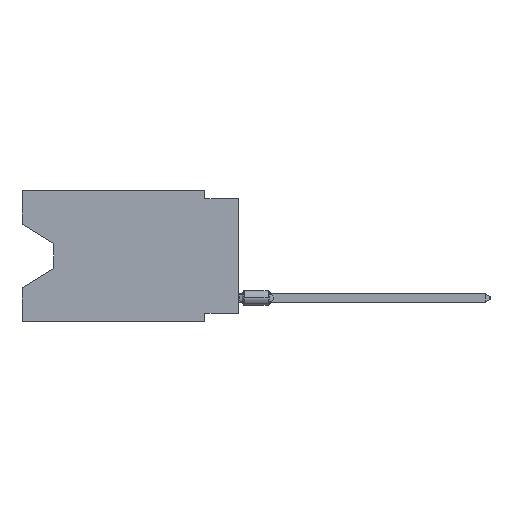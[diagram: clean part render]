
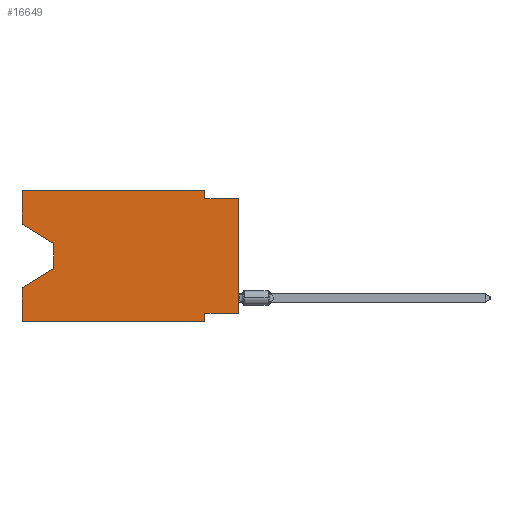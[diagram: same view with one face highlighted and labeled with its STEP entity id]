
A CAD part, left-side view. The second image highlights one B-rep face of the part: STEP entity #16649.
In plain terms, the highlighted planar face has unit normal (-1, 0, 0).
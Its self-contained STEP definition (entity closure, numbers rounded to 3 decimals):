
#107 = VERTEX_POINT ( 'NONE', #27007 ) ;
#235 = LINE ( 'NONE', #24681, #61684 ) ;
#474 = DIRECTION ( 'NONE',  ( 1., 0., 0. ) ) ;
#964 = CARTESIAN_POINT ( 'NONE',  ( 0., 0., -9.271 ) ) ;
#1285 = VERTEX_POINT ( 'NONE', #38073 ) ;
#1314 = EDGE_CURVE ( 'NONE', #22827, #63308, #53799, .T. ) ;
#1412 = CARTESIAN_POINT ( 'NONE',  ( 0., 16.383, 0. ) ) ;
#2039 = ORIENTED_EDGE ( 'NONE', *, *, #60994, .T. ) ;
#2714 = VECTOR ( 'NONE', #15578, 1000. ) ;
#4916 = CARTESIAN_POINT ( 'NONE',  ( 0., 0., -9.271 ) ) ;
#5628 = LINE ( 'NONE', #35447, #20235 ) ;
#5804 = ORIENTED_EDGE ( 'NONE', *, *, #1314, .F. ) ;
#6090 = LINE ( 'NONE', #1412, #43253 ) ;
#6978 = LINE ( 'NONE', #964, #58350 ) ;
#8796 = ORIENTED_EDGE ( 'NONE', *, *, #17196, .T. ) ;
#9389 = CARTESIAN_POINT ( 'NONE',  ( 0., 13.97, -4.013 ) ) ;
#9947 = DIRECTION ( 'NONE',  ( 0., 0., 1. ) ) ;
#9989 = DIRECTION ( 'NONE',  ( 0., 0., 1. ) ) ;
#10262 = LINE ( 'NONE', #55491, #43529 ) ;
#10268 = CARTESIAN_POINT ( 'NONE',  ( 0., 16.383, -9.906 ) ) ;
#10879 = CARTESIAN_POINT ( 'NONE',  ( 0., 16.383, -2.546 ) ) ;
#11327 = DIRECTION ( 'NONE',  ( 0., 1., 0. ) ) ;
#11520 = DIRECTION ( 'NONE',  ( 0., 0., -1. ) ) ;
#14663 = DIRECTION ( 'NONE',  ( 0., 0.855, -0.519 ) ) ;
#15171 = ORIENTED_EDGE ( 'NONE', *, *, #45111, .T. ) ;
#15542 = FACE_OUTER_BOUND ( 'NONE', #16884, .T. ) ;
#15578 = DIRECTION ( 'NONE',  ( 0., -0.855, -0.519 ) ) ;
#15787 = EDGE_CURVE ( 'NONE', #16106, #47020, #6978, .T. ) ;
#16106 = VERTEX_POINT ( 'NONE', #4916 ) ;
#16649 = ADVANCED_FACE ( 'NONE', ( #15542 ), #35950, .F. ) ;
#16884 = EDGE_LOOP ( 'NONE', ( #2039, #22891, #30911, #37083, #8796, #61021, #62279, #15171, #5804, #29706, #55651, #22345 ) ) ;
#17196 = EDGE_CURVE ( 'NONE', #1285, #39355, #55821, .T. ) ;
#17197 = EDGE_CURVE ( 'NONE', #65862, #59636, #235, .T. ) ;
#18954 = VECTOR ( 'NONE', #40252, 1000. ) ;
#19120 = LINE ( 'NONE', #29165, #65400 ) ;
#20235 = VECTOR ( 'NONE', #9989, 1000. ) ;
#22345 = ORIENTED_EDGE ( 'NONE', *, *, #27818, .F. ) ;
#22827 = VERTEX_POINT ( 'NONE', #37944 ) ;
#22891 = ORIENTED_EDGE ( 'NONE', *, *, #58795, .T. ) ;
#22984 = CARTESIAN_POINT ( 'NONE',  ( 0., 0., -0.635 ) ) ;
#23336 = CARTESIAN_POINT ( 'NONE',  ( 0., 2.54, 0. ) ) ;
#23475 = DIRECTION ( 'NONE',  ( 0., 0., 1. ) ) ;
#24681 = CARTESIAN_POINT ( 'NONE',  ( 0., 13.97, -5.893 ) ) ;
#25012 = DIRECTION ( 'NONE',  ( 0., -1., 0. ) ) ;
#26496 = DIRECTION ( 'NONE',  ( 0., -1., 0. ) ) ;
#27007 = CARTESIAN_POINT ( 'NONE',  ( 0., 16.383, 0. ) ) ;
#27818 = EDGE_CURVE ( 'NONE', #33491, #107, #5628, .T. ) ;
#29165 = CARTESIAN_POINT ( 'NONE',  ( 0., 0., 0. ) ) ;
#29598 = EDGE_CURVE ( 'NONE', #51158, #22827, #59493, .T. ) ;
#29706 = ORIENTED_EDGE ( 'NONE', *, *, #29598, .F. ) ;
#30911 = ORIENTED_EDGE ( 'NONE', *, *, #17197, .T. ) ;
#31284 = LINE ( 'NONE', #57379, #53816 ) ;
#32179 = CARTESIAN_POINT ( 'NONE',  ( 0., 0., -0.635 ) ) ;
#32704 = CARTESIAN_POINT ( 'NONE',  ( 0., 16.383, -7.36 ) ) ;
#33261 = VECTOR ( 'NONE', #43780, 1000. ) ;
#33491 = VERTEX_POINT ( 'NONE', #43591 ) ;
#33880 = VECTOR ( 'NONE', #25012, 1000. ) ;
#35447 = CARTESIAN_POINT ( 'NONE',  ( 0., 16.383, 0. ) ) ;
#35950 = PLANE ( 'NONE',  #45597 ) ;
#37083 = ORIENTED_EDGE ( 'NONE', *, *, #64034, .F. ) ;
#37892 = VERTEX_POINT ( 'NONE', #9389 ) ;
#37944 = CARTESIAN_POINT ( 'NONE',  ( 0., 2.54, -0.635 ) ) ;
#38073 = CARTESIAN_POINT ( 'NONE',  ( 0., 16.383, -9.906 ) ) ;
#39355 = VERTEX_POINT ( 'NONE', #65131 ) ;
#39934 = CARTESIAN_POINT ( 'NONE',  ( 0., 2.54, -9.906 ) ) ;
#40252 = DIRECTION ( 'NONE',  ( 0., 0., -1. ) ) ;
#41322 = DIRECTION ( 'NONE',  ( 0., 0., -1. ) ) ;
#43253 = VECTOR ( 'NONE', #26496, 1000. ) ;
#43529 = VECTOR ( 'NONE', #9947, 1000. ) ;
#43591 = CARTESIAN_POINT ( 'NONE',  ( 0., 16.383, -2.546 ) ) ;
#43780 = DIRECTION ( 'NONE',  ( 0., 0., -1. ) ) ;
#44616 = LINE ( 'NONE', #39934, #18954 ) ;
#45111 = EDGE_CURVE ( 'NONE', #16106, #63308, #19120, .T. ) ;
#45597 = AXIS2_PLACEMENT_3D ( 'NONE', #46348, #474, #41322 ) ;
#46348 = CARTESIAN_POINT ( 'NONE',  ( 0., 16.383, 0. ) ) ;
#47020 = VERTEX_POINT ( 'NONE', #55108 ) ;
#47716 = VECTOR ( 'NONE', #48451, 1000. ) ;
#48451 = DIRECTION ( 'NONE',  ( 0., -1., 0. ) ) ;
#48663 = CARTESIAN_POINT ( 'NONE',  ( 0., 13.97, -5.893 ) ) ;
#50255 = EDGE_CURVE ( 'NONE', #107, #51158, #6090, .T. ) ;
#51158 = VERTEX_POINT ( 'NONE', #60638 ) ;
#53799 = LINE ( 'NONE', #22984, #47716 ) ;
#53816 = VECTOR ( 'NONE', #11520, 1000. ) ;
#55108 = CARTESIAN_POINT ( 'NONE',  ( 0., 2.54, -9.271 ) ) ;
#55491 = CARTESIAN_POINT ( 'NONE',  ( 0., 16.383, 0. ) ) ;
#55651 = ORIENTED_EDGE ( 'NONE', *, *, #50255, .F. ) ;
#55821 = LINE ( 'NONE', #10268, #33880 ) ;
#57379 = CARTESIAN_POINT ( 'NONE',  ( 0., 13.97, -4.013 ) ) ;
#58350 = VECTOR ( 'NONE', #11327, 1000. ) ;
#58795 = EDGE_CURVE ( 'NONE', #37892, #65862, #31284, .T. ) ;
#59493 = LINE ( 'NONE', #23336, #33261 ) ;
#59636 = VERTEX_POINT ( 'NONE', #32704 ) ;
#60638 = CARTESIAN_POINT ( 'NONE',  ( 0., 2.54, 0. ) ) ;
#60994 = EDGE_CURVE ( 'NONE', #33491, #37892, #65812, .T. ) ;
#61021 = ORIENTED_EDGE ( 'NONE', *, *, #63030, .F. ) ;
#61684 = VECTOR ( 'NONE', #14663, 1000. ) ;
#62279 = ORIENTED_EDGE ( 'NONE', *, *, #15787, .F. ) ;
#63030 = EDGE_CURVE ( 'NONE', #47020, #39355, #44616, .T. ) ;
#63308 = VERTEX_POINT ( 'NONE', #32179 ) ;
#64034 = EDGE_CURVE ( 'NONE', #1285, #59636, #10262, .T. ) ;
#65131 = CARTESIAN_POINT ( 'NONE',  ( 0., 2.54, -9.906 ) ) ;
#65400 = VECTOR ( 'NONE', #23475, 1000. ) ;
#65812 = LINE ( 'NONE', #10879, #2714 ) ;
#65862 = VERTEX_POINT ( 'NONE', #48663 ) ;
